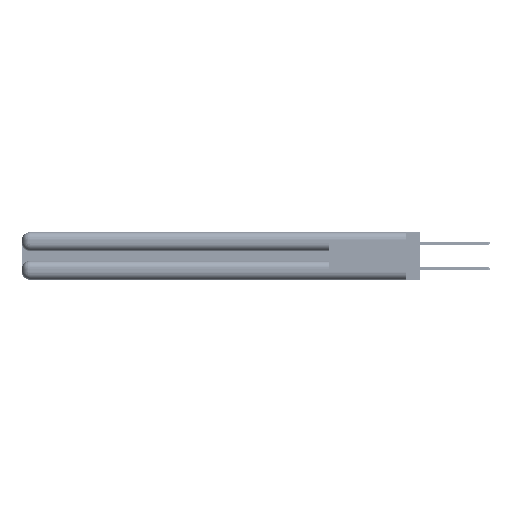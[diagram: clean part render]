
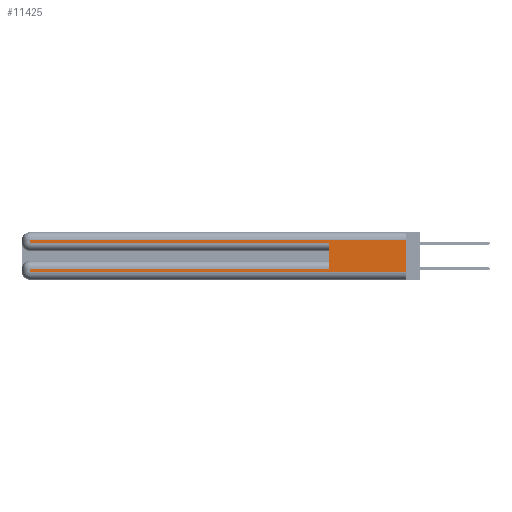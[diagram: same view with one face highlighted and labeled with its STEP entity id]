
A CAD part, left-side view. The second image highlights one B-rep face of the part: STEP entity #11425.
In plain terms, the highlighted planar face has unit normal (-1, 0, 0).
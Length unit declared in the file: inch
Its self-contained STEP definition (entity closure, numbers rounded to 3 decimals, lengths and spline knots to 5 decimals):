
#1642 = CARTESIAN_POINT ( 'NONE',  ( 0., 0.6, 0.145 ) ) ;
#1783 = LINE ( 'NONE', #1642, #49571 ) ;
#4189 = CARTESIAN_POINT ( 'NONE',  ( 0., 0.6, 0.085 ) ) ;
#6687 = PLANE ( 'NONE',  #32216 ) ;
#8366 = VERTEX_POINT ( 'NONE', #4189 ) ;
#9045 = VECTOR ( 'NONE', #18752, 39.37008 ) ;
#9297 = CARTESIAN_POINT ( 'NONE',  ( 0., 2.94, 0.06 ) ) ;
#10350 = VECTOR ( 'NONE', #33310, 39.37008 ) ;
#11341 = VERTEX_POINT ( 'NONE', #42069 ) ;
#11425 = ADVANCED_FACE ( 'NONE', ( #40946 ), #6687, .F. ) ;
#11627 = DIRECTION ( 'NONE',  ( 0., 0., -1. ) ) ;
#12176 = DIRECTION ( 'NONE',  ( 0., -1., 0. ) ) ;
#12634 = CARTESIAN_POINT ( 'NONE',  ( 0., 0., 0.285 ) ) ;
#12874 = ORIENTED_EDGE ( 'NONE', *, *, #37274, .T. ) ;
#13173 = VERTEX_POINT ( 'NONE', #9297 ) ;
#15406 = CARTESIAN_POINT ( 'NONE',  ( 0., 0., 0.085 ) ) ;
#15934 = EDGE_CURVE ( 'NONE', #34023, #52185, #27569, .T. ) ;
#15977 = VECTOR ( 'NONE', #53739, 39.37008 ) ;
#16402 = ORIENTED_EDGE ( 'NONE', *, *, #34626, .T. ) ;
#18470 = EDGE_LOOP ( 'NONE', ( #42298, #24912, #16402, #41288, #53106, #46911, #12874, #25623 ) ) ;
#18752 = DIRECTION ( 'NONE',  ( 0., 0., -1. ) ) ;
#20189 = CARTESIAN_POINT ( 'NONE',  ( 0., 0., 0.37 ) ) ;
#20427 = EDGE_CURVE ( 'NONE', #8366, #11341, #1783, .T. ) ;
#20867 = CARTESIAN_POINT ( 'NONE',  ( 0., 2.94, 0.285 ) ) ;
#22252 = VECTOR ( 'NONE', #12176, 39.37008 ) ;
#23017 = DIRECTION ( 'NONE',  ( 0., 0., 1. ) ) ;
#23727 = VECTOR ( 'NONE', #53945, 39.37008 ) ;
#24912 = ORIENTED_EDGE ( 'NONE', *, *, #15934, .T. ) ;
#25114 = CARTESIAN_POINT ( 'NONE',  ( 0., 0., 0.06 ) ) ;
#25398 = LINE ( 'NONE', #44634, #9045 ) ;
#25623 = ORIENTED_EDGE ( 'NONE', *, *, #38388, .T. ) ;
#27150 = CARTESIAN_POINT ( 'NONE',  ( 0., 2.94, 0.085 ) ) ;
#27569 = LINE ( 'NONE', #28152, #15977 ) ;
#28152 = CARTESIAN_POINT ( 'NONE',  ( 0., 0., 0.31 ) ) ;
#29393 = DIRECTION ( 'NONE',  ( 0., -1., 0. ) ) ;
#30390 = VERTEX_POINT ( 'NONE', #27150 ) ;
#31757 = LINE ( 'NONE', #25114, #22252 ) ;
#31872 = CARTESIAN_POINT ( 'NONE',  ( 0., 0., 0.06 ) ) ;
#32216 = AXIS2_PLACEMENT_3D ( 'NONE', #33329, #37724, #11627 ) ;
#33310 = DIRECTION ( 'NONE',  ( 0., 0., -1. ) ) ;
#33329 = CARTESIAN_POINT ( 'NONE',  ( 0., 0., 0.37 ) ) ;
#33988 = CARTESIAN_POINT ( 'NONE',  ( 0., 2.94, 0.31 ) ) ;
#34023 = VERTEX_POINT ( 'NONE', #39070 ) ;
#34626 = EDGE_CURVE ( 'NONE', #52185, #37431, #25398, .T. ) ;
#36327 = VECTOR ( 'NONE', #29393, 39.37008 ) ;
#36752 = DIRECTION ( 'NONE',  ( 0., 1., 0. ) ) ;
#37274 = EDGE_CURVE ( 'NONE', #30390, #13173, #48947, .T. ) ;
#37281 = EDGE_CURVE ( 'NONE', #8366, #30390, #42763, .T. ) ;
#37431 = VERTEX_POINT ( 'NONE', #20867 ) ;
#37724 = DIRECTION ( 'NONE',  ( 1., 0., 0. ) ) ;
#38388 = EDGE_CURVE ( 'NONE', #13173, #46800, #31757, .T. ) ;
#39070 = CARTESIAN_POINT ( 'NONE',  ( 0., 0., 0.31 ) ) ;
#40946 = FACE_OUTER_BOUND ( 'NONE', #18470, .T. ) ;
#41288 = ORIENTED_EDGE ( 'NONE', *, *, #52748, .T. ) ;
#42069 = CARTESIAN_POINT ( 'NONE',  ( 0., 0.6, 0.285 ) ) ;
#42298 = ORIENTED_EDGE ( 'NONE', *, *, #49434, .F. ) ;
#42763 = LINE ( 'NONE', #15406, #48296 ) ;
#43006 = LINE ( 'NONE', #20189, #10350 ) ;
#44634 = CARTESIAN_POINT ( 'NONE',  ( 0., 2.94, 0.37 ) ) ;
#46552 = LINE ( 'NONE', #12634, #36327 ) ;
#46800 = VERTEX_POINT ( 'NONE', #31872 ) ;
#46911 = ORIENTED_EDGE ( 'NONE', *, *, #37281, .T. ) ;
#48296 = VECTOR ( 'NONE', #36752, 39.37008 ) ;
#48947 = LINE ( 'NONE', #49754, #23727 ) ;
#49434 = EDGE_CURVE ( 'NONE', #34023, #46800, #43006, .T. ) ;
#49571 = VECTOR ( 'NONE', #23017, 39.37008 ) ;
#49754 = CARTESIAN_POINT ( 'NONE',  ( 0., 2.94, 0.37 ) ) ;
#52185 = VERTEX_POINT ( 'NONE', #33988 ) ;
#52748 = EDGE_CURVE ( 'NONE', #37431, #11341, #46552, .T. ) ;
#53106 = ORIENTED_EDGE ( 'NONE', *, *, #20427, .F. ) ;
#53739 = DIRECTION ( 'NONE',  ( 0., 1., 0. ) ) ;
#53945 = DIRECTION ( 'NONE',  ( 0., 0., -1. ) ) ;
